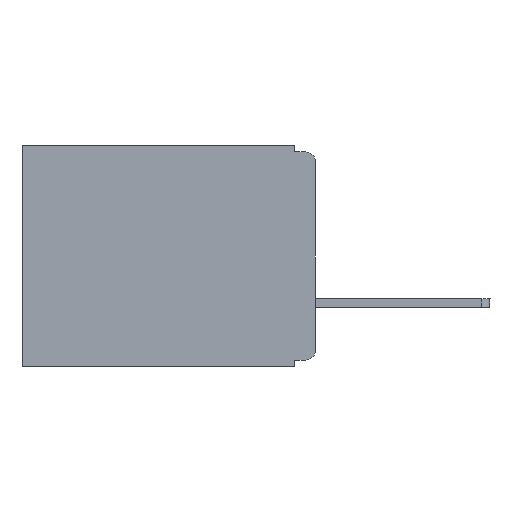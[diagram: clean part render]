
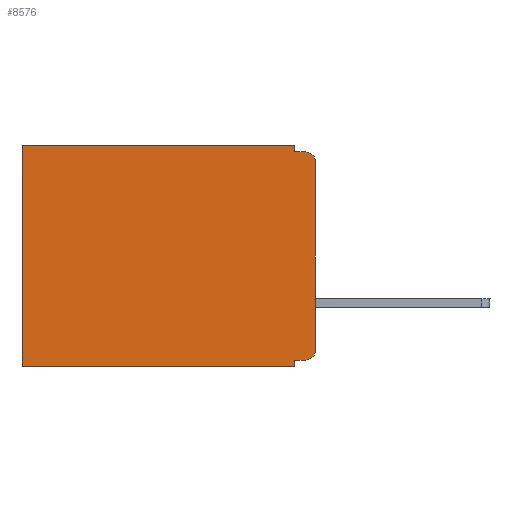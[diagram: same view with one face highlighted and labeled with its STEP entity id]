
A CAD part, left-side view. The second image highlights one B-rep face of the part: STEP entity #8576.
In plain terms, the highlighted planar face has unit normal (-1, 0, 0).
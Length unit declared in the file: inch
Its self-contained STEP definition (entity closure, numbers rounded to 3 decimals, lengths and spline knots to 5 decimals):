
#490 = CARTESIAN_POINT ( 'NONE',  ( 0.3, 0., -0.33 ) ) ;
#525 = DIRECTION ( 'NONE',  ( 0., 0., -1. ) ) ;
#585 = DIRECTION ( 'NONE',  ( 0., 1., 0. ) ) ;
#817 = DIRECTION ( 'NONE',  ( 0., 1., 0. ) ) ;
#841 = DIRECTION ( 'NONE',  ( 0., 0., -1. ) ) ;
#1181 = EDGE_CURVE ( 'NONE', #6070, #3456, #4395, .T. ) ;
#1298 = CARTESIAN_POINT ( 'NONE',  ( 0.3, 0.031, -0.32 ) ) ;
#1547 = CARTESIAN_POINT ( 'NONE',  ( 0.3, 0.031, -0.33 ) ) ;
#1912 = VECTOR ( 'NONE', #841, 39.37008 ) ;
#2141 = VECTOR ( 'NONE', #585, 39.37008 ) ;
#2481 = VERTEX_POINT ( 'NONE', #6226 ) ;
#2643 = CARTESIAN_POINT ( 'NONE',  ( 0.3, 0.437, 0. ) ) ;
#2648 = AXIS2_PLACEMENT_3D ( 'NONE', #13633, #6076, #9317 ) ;
#2718 = ORIENTED_EDGE ( 'NONE', *, *, #4451, .T. ) ;
#2754 = ORIENTED_EDGE ( 'NONE', *, *, #13193, .F. ) ;
#2856 = VECTOR ( 'NONE', #10534, 39.37008 ) ;
#2878 = AXIS2_PLACEMENT_3D ( 'NONE', #12338, #5865, #9209 ) ;
#2899 = VERTEX_POINT ( 'NONE', #10142 ) ;
#2912 = CARTESIAN_POINT ( 'NONE',  ( 0.3, 0.437, -0.33 ) ) ;
#2966 = EDGE_CURVE ( 'NONE', #11795, #3456, #10304, .T. ) ;
#3456 = VERTEX_POINT ( 'NONE', #5279 ) ;
#3480 = CARTESIAN_POINT ( 'NONE',  ( 0.3, 0.015, -0.305 ) ) ;
#3650 = ORIENTED_EDGE ( 'NONE', *, *, #5619, .F. ) ;
#3660 = LINE ( 'NONE', #7328, #2856 ) ;
#4175 = EDGE_CURVE ( 'NONE', #10104, #10097, #5792, .T. ) ;
#4276 = CARTESIAN_POINT ( 'NONE',  ( 0.3, 0.031, 0. ) ) ;
#4370 = LINE ( 'NONE', #490, #6825 ) ;
#4395 = LINE ( 'NONE', #11203, #13003 ) ;
#4451 = EDGE_CURVE ( 'NONE', #11065, #11795, #10767, .T. ) ;
#5200 = VERTEX_POINT ( 'NONE', #6571 ) ;
#5279 = CARTESIAN_POINT ( 'NONE',  ( 0.3, 0.437, -0.33 ) ) ;
#5490 = VECTOR ( 'NONE', #11377, 39.37008 ) ;
#5580 = ORIENTED_EDGE ( 'NONE', *, *, #2966, .T. ) ;
#5598 = EDGE_CURVE ( 'NONE', #10104, #11127, #6405, .T. ) ;
#5619 = EDGE_CURVE ( 'NONE', #2481, #10097, #4370, .T. ) ;
#5792 = CIRCLE ( 'NONE', #5916, 0.015 ) ;
#5865 = DIRECTION ( 'NONE',  ( -1., 0., 0. ) ) ;
#5916 = AXIS2_PLACEMENT_3D ( 'NONE', #3480, #10972, #525 ) ;
#6070 = VERTEX_POINT ( 'NONE', #9282 ) ;
#6076 = DIRECTION ( 'NONE',  ( 1., 0., 0. ) ) ;
#6213 = PLANE ( 'NONE',  #2648 ) ;
#6226 = CARTESIAN_POINT ( 'NONE',  ( 0.3, 0., -0.025 ) ) ;
#6405 = LINE ( 'NONE', #6917, #2141 ) ;
#6571 = CARTESIAN_POINT ( 'NONE',  ( 0.3, 0.015, -0.01 ) ) ;
#6805 = EDGE_CURVE ( 'NONE', #2481, #5200, #12671, .T. ) ;
#6825 = VECTOR ( 'NONE', #8929, 39.37008 ) ;
#6917 = CARTESIAN_POINT ( 'NONE',  ( 0.3, 0., -0.32 ) ) ;
#7328 = CARTESIAN_POINT ( 'NONE',  ( 0.3, 0.031, 0. ) ) ;
#7542 = CARTESIAN_POINT ( 'NONE',  ( 0.3, 0., -0.305 ) ) ;
#7864 = DIRECTION ( 'NONE',  ( 0., -1., 0. ) ) ;
#8031 = DIRECTION ( 'NONE',  ( 0., 1., 0. ) ) ;
#8054 = LINE ( 'NONE', #9950, #11897 ) ;
#8576 = ADVANCED_FACE ( 'NONE', ( #10773 ), #6213, .F. ) ;
#8687 = EDGE_CURVE ( 'NONE', #11065, #2899, #3660, .T. ) ;
#8784 = ORIENTED_EDGE ( 'NONE', *, *, #1181, .F. ) ;
#8929 = DIRECTION ( 'NONE',  ( 0., 0., -1. ) ) ;
#8978 = LINE ( 'NONE', #1547, #5490 ) ;
#9209 = DIRECTION ( 'NONE',  ( 0., 0., -1. ) ) ;
#9282 = CARTESIAN_POINT ( 'NONE',  ( 0.3, 0.031, -0.33 ) ) ;
#9317 = DIRECTION ( 'NONE',  ( 0., 0., -1. ) ) ;
#9762 = VECTOR ( 'NONE', #817, 39.37008 ) ;
#9911 = ORIENTED_EDGE ( 'NONE', *, *, #8687, .F. ) ;
#9950 = CARTESIAN_POINT ( 'NONE',  ( 0.3, 0., -0.01 ) ) ;
#9967 = ORIENTED_EDGE ( 'NONE', *, *, #4175, .T. ) ;
#10097 = VERTEX_POINT ( 'NONE', #7542 ) ;
#10104 = VERTEX_POINT ( 'NONE', #12182 ) ;
#10142 = CARTESIAN_POINT ( 'NONE',  ( 0.3, 0.031, -0.01 ) ) ;
#10304 = LINE ( 'NONE', #2912, #1912 ) ;
#10358 = EDGE_LOOP ( 'NONE', ( #3650, #12181, #12122, #9911, #2718, #5580, #8784, #2754, #12761, #9967 ) ) ;
#10534 = DIRECTION ( 'NONE',  ( 0., 0., -1. ) ) ;
#10767 = LINE ( 'NONE', #12502, #9762 ) ;
#10773 = FACE_OUTER_BOUND ( 'NONE', #10358, .T. ) ;
#10972 = DIRECTION ( 'NONE',  ( -1., 0., 0. ) ) ;
#11065 = VERTEX_POINT ( 'NONE', #4276 ) ;
#11127 = VERTEX_POINT ( 'NONE', #1298 ) ;
#11203 = CARTESIAN_POINT ( 'NONE',  ( 0.3, 0., -0.33 ) ) ;
#11260 = EDGE_CURVE ( 'NONE', #2899, #5200, #8054, .T. ) ;
#11377 = DIRECTION ( 'NONE',  ( 0., 0., -1. ) ) ;
#11795 = VERTEX_POINT ( 'NONE', #2643 ) ;
#11897 = VECTOR ( 'NONE', #7864, 39.37008 ) ;
#12122 = ORIENTED_EDGE ( 'NONE', *, *, #11260, .F. ) ;
#12181 = ORIENTED_EDGE ( 'NONE', *, *, #6805, .T. ) ;
#12182 = CARTESIAN_POINT ( 'NONE',  ( 0.3, 0.015, -0.32 ) ) ;
#12338 = CARTESIAN_POINT ( 'NONE',  ( 0.3, 0.015, -0.025 ) ) ;
#12502 = CARTESIAN_POINT ( 'NONE',  ( 0.3, 0., 0. ) ) ;
#12671 = CIRCLE ( 'NONE', #2878, 0.015 ) ;
#12761 = ORIENTED_EDGE ( 'NONE', *, *, #5598, .F. ) ;
#13003 = VECTOR ( 'NONE', #8031, 39.37008 ) ;
#13193 = EDGE_CURVE ( 'NONE', #11127, #6070, #8978, .T. ) ;
#13633 = CARTESIAN_POINT ( 'NONE',  ( 0.3, 0., -0.33 ) ) ;
